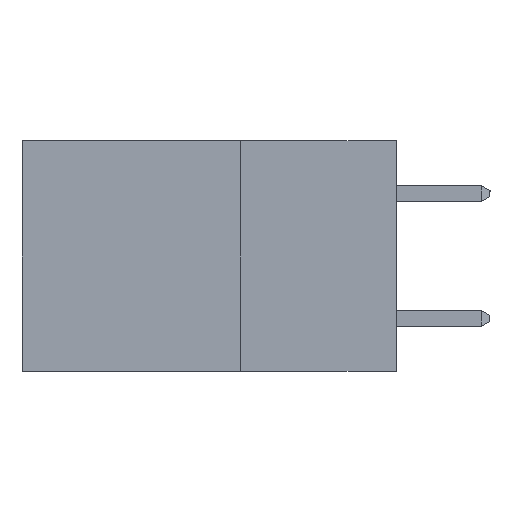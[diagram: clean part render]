
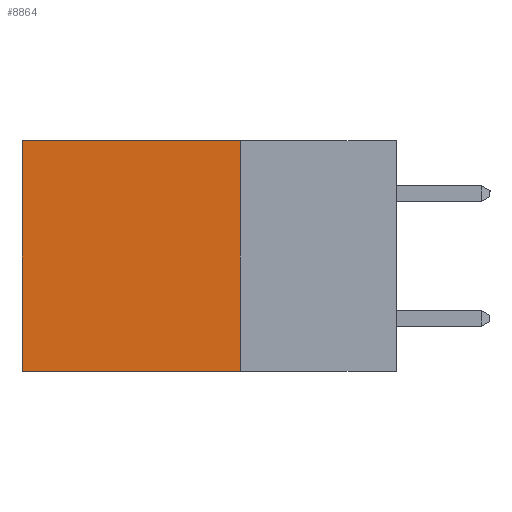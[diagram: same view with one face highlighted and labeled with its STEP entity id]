
A CAD part, left-side view. The second image highlights one B-rep face of the part: STEP entity #8864.
In plain terms, the highlighted planar face has unit normal (-1, 0, 0).
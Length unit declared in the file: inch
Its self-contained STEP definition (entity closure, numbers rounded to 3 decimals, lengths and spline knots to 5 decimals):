
#1309 = DIRECTION ( 'NONE',  ( 0., 0., -1. ) ) ;
#2623 = EDGE_LOOP ( 'NONE', ( #16557, #23063, #12471, #21671 ) ) ;
#3107 = LINE ( 'NONE', #16502, #16797 ) ;
#3742 = CARTESIAN_POINT ( 'NONE',  ( 0.2615, 0.25, -0.37 ) ) ;
#4020 = CARTESIAN_POINT ( 'NONE',  ( 0.2615, 0.6, -0.37 ) ) ;
#4137 = LINE ( 'NONE', #9500, #4774 ) ;
#4214 = CARTESIAN_POINT ( 'NONE',  ( 0.2615, 0.25, -0.37 ) ) ;
#4774 = VECTOR ( 'NONE', #20812, 39.37008 ) ;
#5068 = EDGE_CURVE ( 'NONE', #10550, #12090, #4137, .T. ) ;
#5502 = LINE ( 'NONE', #11110, #15632 ) ;
#7257 = AXIS2_PLACEMENT_3D ( 'NONE', #3742, #11180, #11055 ) ;
#8864 = ADVANCED_FACE ( 'NONE', ( #18350 ), #15054, .F. ) ;
#9500 = CARTESIAN_POINT ( 'NONE',  ( 0.2615, 0.25, -0.37 ) ) ;
#9581 = LINE ( 'NONE', #4214, #14065 ) ;
#10030 = CARTESIAN_POINT ( 'NONE',  ( 0.2615, 0.6, 0. ) ) ;
#10550 = VERTEX_POINT ( 'NONE', #17736 ) ;
#10985 = CARTESIAN_POINT ( 'NONE',  ( 0.2615, 0.25, -0.37 ) ) ;
#11055 = DIRECTION ( 'NONE',  ( 0., 0., -1. ) ) ;
#11110 = CARTESIAN_POINT ( 'NONE',  ( 0.2615, 0.25, 0. ) ) ;
#11180 = DIRECTION ( 'NONE',  ( 1., 0., 0. ) ) ;
#12090 = VERTEX_POINT ( 'NONE', #10985 ) ;
#12471 = ORIENTED_EDGE ( 'NONE', *, *, #5068, .F. ) ;
#13261 = VERTEX_POINT ( 'NONE', #10030 ) ;
#13528 = EDGE_CURVE ( 'NONE', #10550, #13261, #5502, .T. ) ;
#14065 = VECTOR ( 'NONE', #18942, 39.37008 ) ;
#15054 = PLANE ( 'NONE',  #7257 ) ;
#15632 = VECTOR ( 'NONE', #18531, 39.37008 ) ;
#16502 = CARTESIAN_POINT ( 'NONE',  ( 0.2615, 0.6, -0.37 ) ) ;
#16557 = ORIENTED_EDGE ( 'NONE', *, *, #19277, .T. ) ;
#16797 = VECTOR ( 'NONE', #1309, 39.37008 ) ;
#17406 = VERTEX_POINT ( 'NONE', #4020 ) ;
#17736 = CARTESIAN_POINT ( 'NONE',  ( 0.2615, 0.25, 0. ) ) ;
#18350 = FACE_OUTER_BOUND ( 'NONE', #2623, .T. ) ;
#18531 = DIRECTION ( 'NONE',  ( 0., 1., 0. ) ) ;
#18942 = DIRECTION ( 'NONE',  ( 0., 1., 0. ) ) ;
#19277 = EDGE_CURVE ( 'NONE', #13261, #17406, #3107, .T. ) ;
#20028 = EDGE_CURVE ( 'NONE', #12090, #17406, #9581, .T. ) ;
#20812 = DIRECTION ( 'NONE',  ( 0., 0., -1. ) ) ;
#21671 = ORIENTED_EDGE ( 'NONE', *, *, #13528, .T. ) ;
#23063 = ORIENTED_EDGE ( 'NONE', *, *, #20028, .F. ) ;
